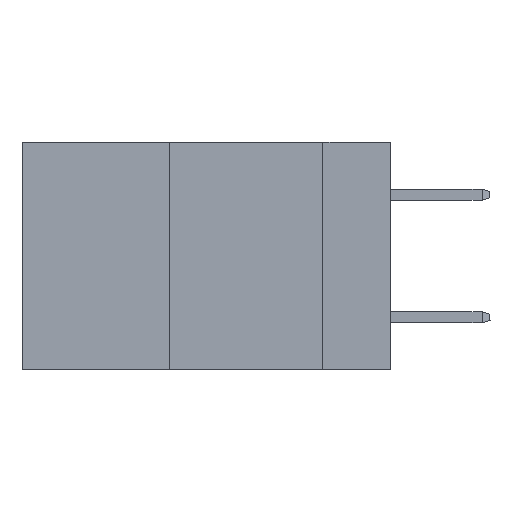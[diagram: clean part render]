
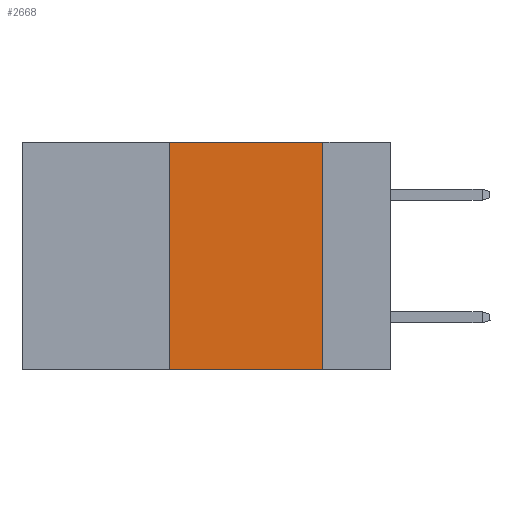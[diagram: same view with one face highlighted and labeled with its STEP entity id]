
A CAD part, left-side view. The second image highlights one B-rep face of the part: STEP entity #2668.
In plain terms, the highlighted planar face has unit normal (-1, 0, 0).
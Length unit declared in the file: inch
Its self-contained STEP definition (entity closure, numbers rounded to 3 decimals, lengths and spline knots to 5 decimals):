
#576 = AXIS2_PLACEMENT_3D ( 'NONE', #12693, #20192, #7898 ) ;
#2427 = VECTOR ( 'NONE', #15070, 39.37008 ) ;
#2668 = ADVANCED_FACE ( 'NONE', ( #15856 ), #15831, .F. ) ;
#3276 = LINE ( 'NONE', #3277, #11470 ) ;
#3277 = CARTESIAN_POINT ( 'NONE',  ( 0., 0.36, 0. ) ) ;
#4641 = EDGE_CURVE ( 'NONE', #6228, #22014, #19167, .T. ) ;
#5548 = ORIENTED_EDGE ( 'NONE', *, *, #4641, .F. ) ;
#6228 = VERTEX_POINT ( 'NONE', #9406 ) ;
#7265 = VECTOR ( 'NONE', #7623, 39.37008 ) ;
#7416 = CARTESIAN_POINT ( 'NONE',  ( 0., 0.36, -0.37 ) ) ;
#7623 = DIRECTION ( 'NONE',  ( 0., -1., 0. ) ) ;
#7898 = DIRECTION ( 'NONE',  ( 0., 0., -1. ) ) ;
#8406 = ORIENTED_EDGE ( 'NONE', *, *, #20640, .F. ) ;
#9406 = CARTESIAN_POINT ( 'NONE',  ( 0., 0.36, 0. ) ) ;
#10694 = CARTESIAN_POINT ( 'NONE',  ( 0., 0.11, -0.37 ) ) ;
#11470 = VECTOR ( 'NONE', #13705, 39.37008 ) ;
#12491 = EDGE_LOOP ( 'NONE', ( #8406, #5548, #15983, #22672 ) ) ;
#12687 = VERTEX_POINT ( 'NONE', #7416 ) ;
#12693 = CARTESIAN_POINT ( 'NONE',  ( 0., 0.6, 0. ) ) ;
#13213 = EDGE_CURVE ( 'NONE', #12687, #6228, #3276, .T. ) ;
#13705 = DIRECTION ( 'NONE',  ( 0., 0., 1. ) ) ;
#15070 = DIRECTION ( 'NONE',  ( 0., 0., -1. ) ) ;
#15586 = LINE ( 'NONE', #17414, #19289 ) ;
#15633 = CARTESIAN_POINT ( 'NONE',  ( 0., 0.11, 0. ) ) ;
#15831 = PLANE ( 'NONE',  #576 ) ;
#15856 = FACE_OUTER_BOUND ( 'NONE', #12491, .T. ) ;
#15973 = LINE ( 'NONE', #15633, #2427 ) ;
#15983 = ORIENTED_EDGE ( 'NONE', *, *, #13213, .F. ) ;
#16369 = CARTESIAN_POINT ( 'NONE',  ( 0., 0.11, 0. ) ) ;
#17107 = VERTEX_POINT ( 'NONE', #10694 ) ;
#17414 = CARTESIAN_POINT ( 'NONE',  ( 0., 0.6, -0.37 ) ) ;
#17477 = DIRECTION ( 'NONE',  ( 0., -1., 0. ) ) ;
#19167 = LINE ( 'NONE', #22591, #7265 ) ;
#19289 = VECTOR ( 'NONE', #17477, 39.37008 ) ;
#20192 = DIRECTION ( 'NONE',  ( 1., 0., 0. ) ) ;
#20640 = EDGE_CURVE ( 'NONE', #22014, #17107, #15973, .T. ) ;
#22014 = VERTEX_POINT ( 'NONE', #16369 ) ;
#22591 = CARTESIAN_POINT ( 'NONE',  ( 0., 0.6, 0. ) ) ;
#22607 = EDGE_CURVE ( 'NONE', #12687, #17107, #15586, .T. ) ;
#22672 = ORIENTED_EDGE ( 'NONE', *, *, #22607, .T. ) ;
